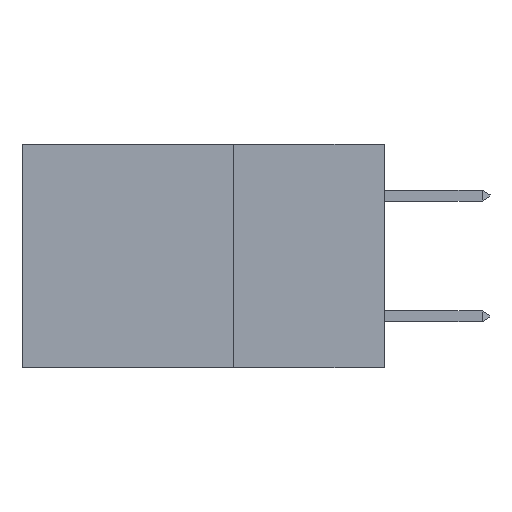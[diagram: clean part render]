
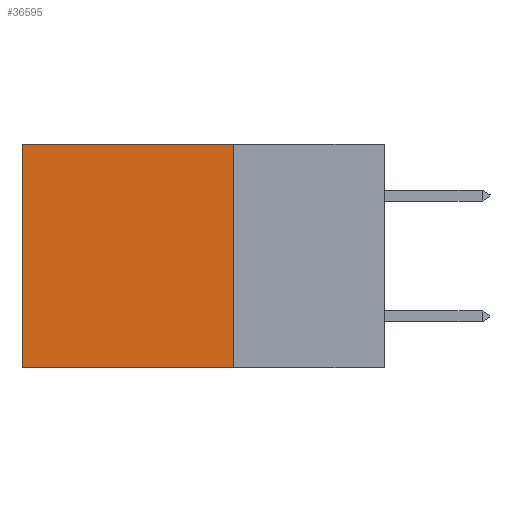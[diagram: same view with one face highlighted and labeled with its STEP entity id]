
A CAD part, left-side view. The second image highlights one B-rep face of the part: STEP entity #36595.
In plain terms, the highlighted planar face has unit normal (-1, 0, 0).
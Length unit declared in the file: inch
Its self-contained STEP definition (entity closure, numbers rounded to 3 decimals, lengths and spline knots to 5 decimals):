
#1059 = VERTEX_POINT ( 'NONE', #25266 ) ;
#3533 = EDGE_CURVE ( 'NONE', #20903, #33049, #20257, .T. ) ;
#3969 = CARTESIAN_POINT ( 'NONE',  ( 0.2875, 0.25, -0.37 ) ) ;
#4366 = DIRECTION ( 'NONE',  ( 0., 0., -1. ) ) ;
#4536 = CARTESIAN_POINT ( 'NONE',  ( 0.2875, 0.25, 0. ) ) ;
#6314 = ORIENTED_EDGE ( 'NONE', *, *, #15554, .F. ) ;
#6363 = VERTEX_POINT ( 'NONE', #3969 ) ;
#6660 = CARTESIAN_POINT ( 'NONE',  ( 0.2875, 0.25, 0. ) ) ;
#7905 = LINE ( 'NONE', #31445, #43168 ) ;
#7961 = EDGE_LOOP ( 'NONE', ( #36153, #14955, #6314, #40445 ) ) ;
#8672 = CARTESIAN_POINT ( 'NONE',  ( 0.2875, 0.6, 0. ) ) ;
#8998 = VECTOR ( 'NONE', #26169, 39.37008 ) ;
#9730 = DIRECTION ( 'NONE',  ( 0., 0., -1. ) ) ;
#10115 = AXIS2_PLACEMENT_3D ( 'NONE', #14809, #35574, #4366 ) ;
#11551 = DIRECTION ( 'NONE',  ( 0., 0., -1. ) ) ;
#14809 = CARTESIAN_POINT ( 'NONE',  ( 0.2875, 0.25, 0. ) ) ;
#14955 = ORIENTED_EDGE ( 'NONE', *, *, #34719, .F. ) ;
#15554 = EDGE_CURVE ( 'NONE', #20903, #6363, #36212, .T. ) ;
#20257 = LINE ( 'NONE', #25886, #8998 ) ;
#20903 = VERTEX_POINT ( 'NONE', #6660 ) ;
#21541 = PLANE ( 'NONE',  #10115 ) ;
#25266 = CARTESIAN_POINT ( 'NONE',  ( 0.2875, 0.6, -0.37 ) ) ;
#25886 = CARTESIAN_POINT ( 'NONE',  ( 0.2875, 0.25, 0. ) ) ;
#26169 = DIRECTION ( 'NONE',  ( 0., 1., 0. ) ) ;
#26915 = EDGE_CURVE ( 'NONE', #33049, #1059, #36976, .T. ) ;
#28219 = VECTOR ( 'NONE', #11551, 39.37008 ) ;
#30029 = VECTOR ( 'NONE', #9730, 39.37008 ) ;
#30966 = FACE_OUTER_BOUND ( 'NONE', #7961, .T. ) ;
#31445 = CARTESIAN_POINT ( 'NONE',  ( 0.2875, 0.25, -0.37 ) ) ;
#33049 = VERTEX_POINT ( 'NONE', #8672 ) ;
#33951 = CARTESIAN_POINT ( 'NONE',  ( 0.2875, 0.6, 0. ) ) ;
#34719 = EDGE_CURVE ( 'NONE', #6363, #1059, #7905, .T. ) ;
#35574 = DIRECTION ( 'NONE',  ( 1., 0., 0. ) ) ;
#36153 = ORIENTED_EDGE ( 'NONE', *, *, #26915, .T. ) ;
#36212 = LINE ( 'NONE', #4536, #28219 ) ;
#36595 = ADVANCED_FACE ( 'NONE', ( #30966 ), #21541, .F. ) ;
#36976 = LINE ( 'NONE', #33951, #30029 ) ;
#38130 = DIRECTION ( 'NONE',  ( 0., 1., 0. ) ) ;
#40445 = ORIENTED_EDGE ( 'NONE', *, *, #3533, .T. ) ;
#43168 = VECTOR ( 'NONE', #38130, 39.37008 ) ;
